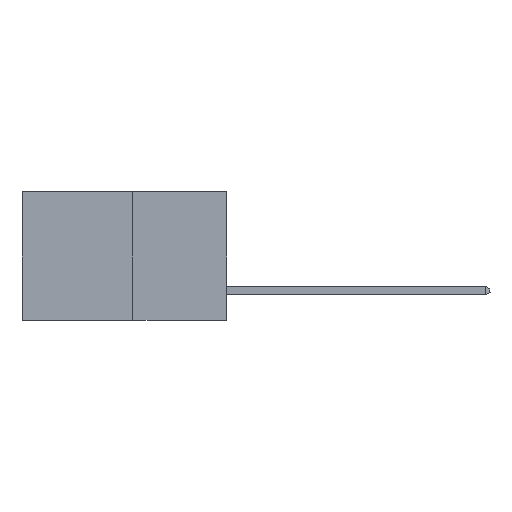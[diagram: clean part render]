
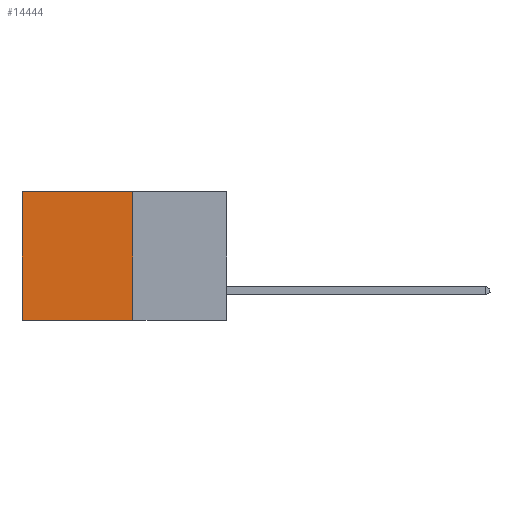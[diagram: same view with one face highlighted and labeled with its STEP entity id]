
A CAD part, left-side view. The second image highlights one B-rep face of the part: STEP entity #14444.
In plain terms, the highlighted planar face has unit normal (-1, 0, 0).
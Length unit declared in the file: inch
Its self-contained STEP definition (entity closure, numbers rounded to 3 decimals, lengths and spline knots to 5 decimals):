
#460 = VERTEX_POINT ( 'NONE', #11591 ) ;
#645 = CARTESIAN_POINT ( 'NONE',  ( 0.277, 0.27, -0.37 ) ) ;
#663 = VERTEX_POINT ( 'NONE', #11186 ) ;
#1107 = LINE ( 'NONE', #10486, #17463 ) ;
#1736 = EDGE_CURVE ( 'NONE', #460, #17919, #5754, .T. ) ;
#2176 = LINE ( 'NONE', #10336, #9839 ) ;
#3876 = CARTESIAN_POINT ( 'NONE',  ( 0.277, 0.27, -0.37 ) ) ;
#4913 = ORIENTED_EDGE ( 'NONE', *, *, #10242, .T. ) ;
#5401 = DIRECTION ( 'NONE',  ( 0., 0., -1. ) ) ;
#5754 = LINE ( 'NONE', #11265, #13877 ) ;
#5895 = DIRECTION ( 'NONE',  ( 0., 0., -1. ) ) ;
#5925 = DIRECTION ( 'NONE',  ( 0., 0., -1. ) ) ;
#6070 = FACE_OUTER_BOUND ( 'NONE', #12665, .T. ) ;
#6367 = ORIENTED_EDGE ( 'NONE', *, *, #1736, .F. ) ;
#8033 = EDGE_CURVE ( 'NONE', #17919, #15637, #1107, .T. ) ;
#9544 = VECTOR ( 'NONE', #18147, 39.37008 ) ;
#9839 = VECTOR ( 'NONE', #5895, 39.37008 ) ;
#10242 = EDGE_CURVE ( 'NONE', #663, #15637, #2176, .T. ) ;
#10336 = CARTESIAN_POINT ( 'NONE',  ( 0.277, 0.59, -0.37 ) ) ;
#10456 = DIRECTION ( 'NONE',  ( 0., 1., 0. ) ) ;
#10486 = CARTESIAN_POINT ( 'NONE',  ( 0.277, 0.27, -0.37 ) ) ;
#11186 = CARTESIAN_POINT ( 'NONE',  ( 0.277, 0.59, 0. ) ) ;
#11265 = CARTESIAN_POINT ( 'NONE',  ( 0.277, 0.27, -0.37 ) ) ;
#11591 = CARTESIAN_POINT ( 'NONE',  ( 0.277, 0.27, 0. ) ) ;
#11797 = EDGE_CURVE ( 'NONE', #460, #663, #12606, .T. ) ;
#11828 = ORIENTED_EDGE ( 'NONE', *, *, #11797, .T. ) ;
#12606 = LINE ( 'NONE', #15118, #9544 ) ;
#12665 = EDGE_LOOP ( 'NONE', ( #4913, #18198, #6367, #11828 ) ) ;
#13877 = VECTOR ( 'NONE', #5925, 39.37008 ) ;
#14444 = ADVANCED_FACE ( 'NONE', ( #6070 ), #19222, .F. ) ;
#14583 = DIRECTION ( 'NONE',  ( 1., 0., 0. ) ) ;
#15118 = CARTESIAN_POINT ( 'NONE',  ( 0.277, 0.27, 0. ) ) ;
#15637 = VERTEX_POINT ( 'NONE', #15729 ) ;
#15729 = CARTESIAN_POINT ( 'NONE',  ( 0.277, 0.59, -0.37 ) ) ;
#17463 = VECTOR ( 'NONE', #10456, 39.37008 ) ;
#17919 = VERTEX_POINT ( 'NONE', #645 ) ;
#18147 = DIRECTION ( 'NONE',  ( 0., 1., 0. ) ) ;
#18198 = ORIENTED_EDGE ( 'NONE', *, *, #8033, .F. ) ;
#19222 = PLANE ( 'NONE',  #19352 ) ;
#19352 = AXIS2_PLACEMENT_3D ( 'NONE', #3876, #14583, #5401 ) ;
